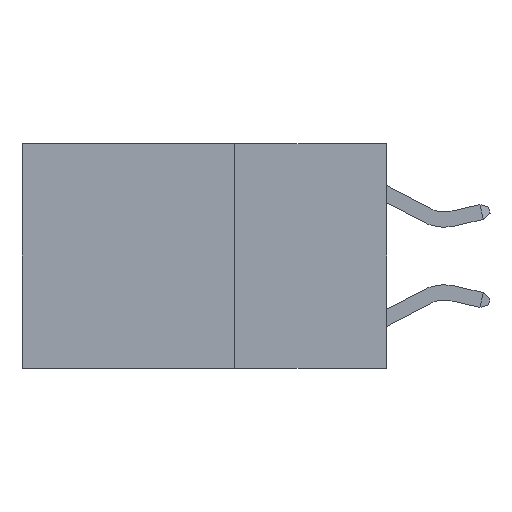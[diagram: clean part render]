
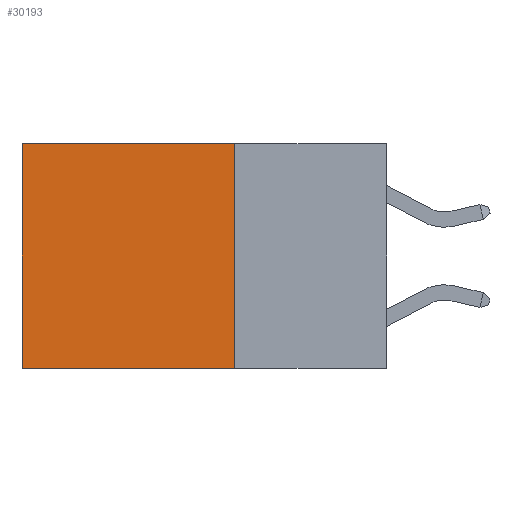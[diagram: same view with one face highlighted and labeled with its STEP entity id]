
A CAD part, left-side view. The second image highlights one B-rep face of the part: STEP entity #30193.
In plain terms, the highlighted planar face has unit normal (-1, 0, 0).
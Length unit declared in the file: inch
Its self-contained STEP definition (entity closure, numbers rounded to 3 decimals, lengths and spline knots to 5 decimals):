
#1134 = EDGE_CURVE ( 'NONE', #22139, #19753, #27416, .T. ) ;
#1970 = PLANE ( 'NONE',  #25536 ) ;
#3821 = DIRECTION ( 'NONE',  ( 0., 0., -1. ) ) ;
#3985 = VECTOR ( 'NONE', #5151, 39.37008 ) ;
#4111 = VERTEX_POINT ( 'NONE', #6858 ) ;
#5151 = DIRECTION ( 'NONE',  ( 0., 0., -1. ) ) ;
#5378 = ORIENTED_EDGE ( 'NONE', *, *, #24749, .T. ) ;
#5740 = EDGE_CURVE ( 'NONE', #19753, #4111, #31688, .T. ) ;
#6858 = CARTESIAN_POINT ( 'NONE',  ( 0.2625, 0.6, -0.37 ) ) ;
#6968 = CARTESIAN_POINT ( 'NONE',  ( 0.2625, 0.6, 0. ) ) ;
#9445 = DIRECTION ( 'NONE',  ( 0., 1., 0. ) ) ;
#10135 = VERTEX_POINT ( 'NONE', #6968 ) ;
#12749 = CARTESIAN_POINT ( 'NONE',  ( 0.2625, 0.25, 0. ) ) ;
#14610 = VECTOR ( 'NONE', #31914, 39.37008 ) ;
#15178 = DIRECTION ( 'NONE',  ( 1., 0., 0. ) ) ;
#17383 = LINE ( 'NONE', #32131, #14610 ) ;
#17385 = ORIENTED_EDGE ( 'NONE', *, *, #1134, .F. ) ;
#17661 = EDGE_CURVE ( 'NONE', #10135, #4111, #29049, .T. ) ;
#19753 = VERTEX_POINT ( 'NONE', #27046 ) ;
#20162 = DIRECTION ( 'NONE',  ( 0., 0., -1. ) ) ;
#21367 = CARTESIAN_POINT ( 'NONE',  ( 0.2625, 0.25, 0. ) ) ;
#21417 = VECTOR ( 'NONE', #3821, 39.37008 ) ;
#22139 = VERTEX_POINT ( 'NONE', #26655 ) ;
#22507 = FACE_OUTER_BOUND ( 'NONE', #24760, .T. ) ;
#22749 = ORIENTED_EDGE ( 'NONE', *, *, #17661, .T. ) ;
#24749 = EDGE_CURVE ( 'NONE', #22139, #10135, #17383, .T. ) ;
#24760 = EDGE_LOOP ( 'NONE', ( #22749, #26685, #17385, #5378 ) ) ;
#25536 = AXIS2_PLACEMENT_3D ( 'NONE', #12749, #15178, #20162 ) ;
#26655 = CARTESIAN_POINT ( 'NONE',  ( 0.2625, 0.25, 0. ) ) ;
#26685 = ORIENTED_EDGE ( 'NONE', *, *, #5740, .F. ) ;
#27046 = CARTESIAN_POINT ( 'NONE',  ( 0.2625, 0.25, -0.37 ) ) ;
#27416 = LINE ( 'NONE', #21367, #21417 ) ;
#29049 = LINE ( 'NONE', #30286, #3985 ) ;
#30193 = ADVANCED_FACE ( 'NONE', ( #22507 ), #1970, .F. ) ;
#30286 = CARTESIAN_POINT ( 'NONE',  ( 0.2625, 0.6, 0. ) ) ;
#31688 = LINE ( 'NONE', #31834, #32922 ) ;
#31834 = CARTESIAN_POINT ( 'NONE',  ( 0.2625, 0.25, -0.37 ) ) ;
#31914 = DIRECTION ( 'NONE',  ( 0., 1., 0. ) ) ;
#32131 = CARTESIAN_POINT ( 'NONE',  ( 0.2625, 0.25, 0. ) ) ;
#32922 = VECTOR ( 'NONE', #9445, 39.37008 ) ;
